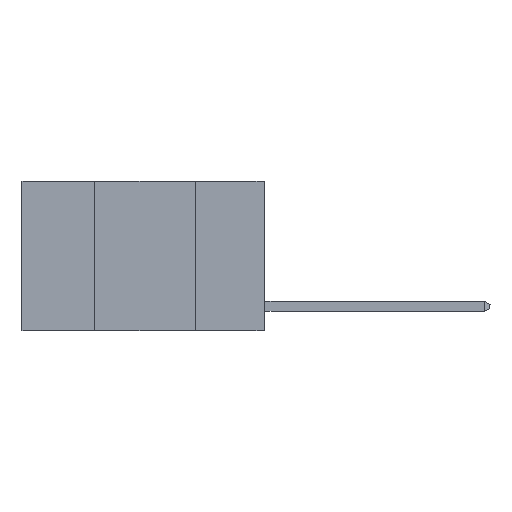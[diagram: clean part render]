
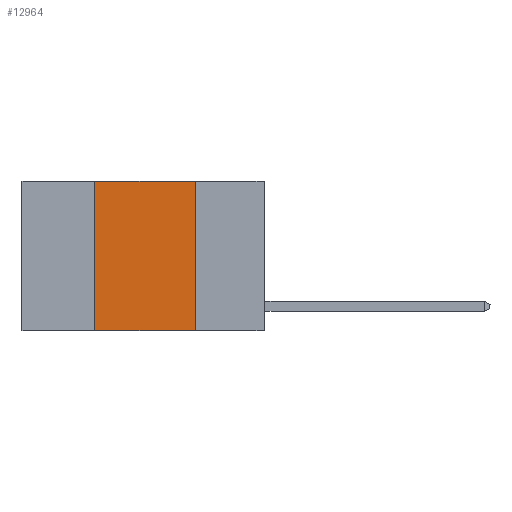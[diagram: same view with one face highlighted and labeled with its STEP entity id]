
A CAD part, left-side view. The second image highlights one B-rep face of the part: STEP entity #12964.
In plain terms, the highlighted planar face has unit normal (-1, 0, 0).
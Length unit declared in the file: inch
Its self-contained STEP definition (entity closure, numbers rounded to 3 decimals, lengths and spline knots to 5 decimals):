
#85 = DIRECTION ( 'NONE',  ( 0., -1., 0. ) ) ;
#185 = CARTESIAN_POINT ( 'NONE',  ( 0., 0.42, 0. ) ) ;
#913 = VECTOR ( 'NONE', #9051, 39.37008 ) ;
#1302 = LINE ( 'NONE', #5224, #5245 ) ;
#1699 = LINE ( 'NONE', #185, #913 ) ;
#2128 = CARTESIAN_POINT ( 'NONE',  ( 0., 0.6, -0.37 ) ) ;
#2574 = CARTESIAN_POINT ( 'NONE',  ( 0., 0.6, 0. ) ) ;
#2598 = ORIENTED_EDGE ( 'NONE', *, *, #16027, .T. ) ;
#2677 = DIRECTION ( 'NONE',  ( 0., 0., -1. ) ) ;
#3357 = AXIS2_PLACEMENT_3D ( 'NONE', #2574, #12734, #2677 ) ;
#3359 = VERTEX_POINT ( 'NONE', #4464 ) ;
#4019 = EDGE_CURVE ( 'NONE', #3359, #12616, #16483, .T. ) ;
#4430 = EDGE_CURVE ( 'NONE', #13867, #4986, #1699, .T. ) ;
#4464 = CARTESIAN_POINT ( 'NONE',  ( 0., 0.17, 0. ) ) ;
#4601 = DIRECTION ( 'NONE',  ( 0., 0., -1. ) ) ;
#4906 = ORIENTED_EDGE ( 'NONE', *, *, #4019, .F. ) ;
#4986 = VERTEX_POINT ( 'NONE', #14005 ) ;
#5224 = CARTESIAN_POINT ( 'NONE',  ( 0., 0.6, 0. ) ) ;
#5245 = VECTOR ( 'NONE', #85, 39.37008 ) ;
#6273 = FACE_OUTER_BOUND ( 'NONE', #9587, .T. ) ;
#6358 = ORIENTED_EDGE ( 'NONE', *, *, #4430, .F. ) ;
#7183 = CARTESIAN_POINT ( 'NONE',  ( 0., 0.17, 0. ) ) ;
#8170 = EDGE_CURVE ( 'NONE', #4986, #3359, #1302, .T. ) ;
#8457 = ORIENTED_EDGE ( 'NONE', *, *, #8170, .F. ) ;
#8485 = VECTOR ( 'NONE', #4601, 39.37008 ) ;
#9051 = DIRECTION ( 'NONE',  ( 0., 0., 1. ) ) ;
#9587 = EDGE_LOOP ( 'NONE', ( #4906, #8457, #6358, #2598 ) ) ;
#10979 = DIRECTION ( 'NONE',  ( 0., -1., 0. ) ) ;
#12616 = VERTEX_POINT ( 'NONE', #12717 ) ;
#12717 = CARTESIAN_POINT ( 'NONE',  ( 0., 0.17, -0.37 ) ) ;
#12734 = DIRECTION ( 'NONE',  ( 1., 0., 0. ) ) ;
#12964 = ADVANCED_FACE ( 'NONE', ( #6273 ), #16400, .F. ) ;
#13693 = CARTESIAN_POINT ( 'NONE',  ( 0., 0.42, -0.37 ) ) ;
#13818 = LINE ( 'NONE', #2128, #15836 ) ;
#13867 = VERTEX_POINT ( 'NONE', #13693 ) ;
#14005 = CARTESIAN_POINT ( 'NONE',  ( 0., 0.42, 0. ) ) ;
#15836 = VECTOR ( 'NONE', #10979, 39.37008 ) ;
#16027 = EDGE_CURVE ( 'NONE', #13867, #12616, #13818, .T. ) ;
#16400 = PLANE ( 'NONE',  #3357 ) ;
#16483 = LINE ( 'NONE', #7183, #8485 ) ;
